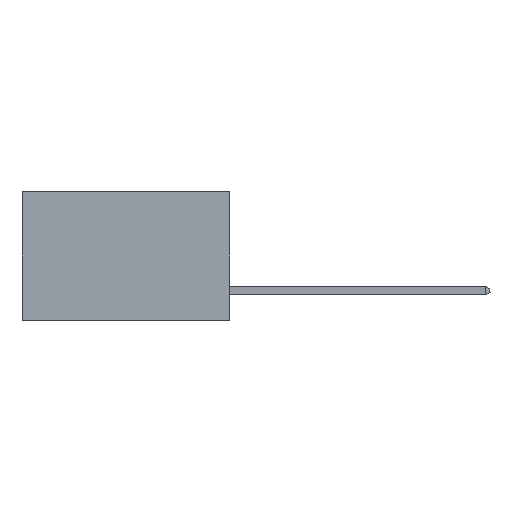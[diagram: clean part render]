
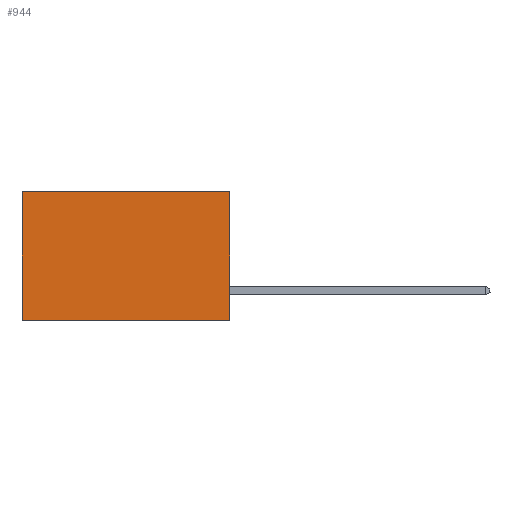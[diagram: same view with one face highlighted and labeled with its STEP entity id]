
A CAD part, left-side view. The second image highlights one B-rep face of the part: STEP entity #944.
In plain terms, the highlighted planar face has unit normal (-1, 0, 0).
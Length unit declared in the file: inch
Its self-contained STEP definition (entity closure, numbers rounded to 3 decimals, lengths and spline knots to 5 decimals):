
#235 = FACE_OUTER_BOUND ( 'NONE', #9415, .T. ) ;
#944 = ADVANCED_FACE ( 'NONE', ( #235 ), #9784, .F. ) ;
#2129 = VECTOR ( 'NONE', #9009, 39.37008 ) ;
#2631 = CARTESIAN_POINT ( 'NONE',  ( 0.298, 0., 0. ) ) ;
#3233 = ORIENTED_EDGE ( 'NONE', *, *, #7428, .F. ) ;
#3327 = VECTOR ( 'NONE', #15590, 39.37008 ) ;
#4082 = DIRECTION ( 'NONE',  ( 0., 1., 0. ) ) ;
#4445 = ORIENTED_EDGE ( 'NONE', *, *, #4800, .F. ) ;
#4634 = LINE ( 'NONE', #8909, #10448 ) ;
#4759 = VERTEX_POINT ( 'NONE', #16366 ) ;
#4800 = EDGE_CURVE ( 'NONE', #4759, #13359, #9547, .T. ) ;
#5524 = DIRECTION ( 'NONE',  ( 1., 0., 0. ) ) ;
#6224 = CARTESIAN_POINT ( 'NONE',  ( 0.298, 0.6, 0. ) ) ;
#7428 = EDGE_CURVE ( 'NONE', #13359, #11709, #4634, .T. ) ;
#7526 = VECTOR ( 'NONE', #4082, 39.37008 ) ;
#8736 = DIRECTION ( 'NONE',  ( 0., 1., 0. ) ) ;
#8909 = CARTESIAN_POINT ( 'NONE',  ( 0.298, 0., -0.37 ) ) ;
#9009 = DIRECTION ( 'NONE',  ( 0., 0., -1. ) ) ;
#9016 = CARTESIAN_POINT ( 'NONE',  ( 0.298, 0.6, -0.37 ) ) ;
#9415 = EDGE_LOOP ( 'NONE', ( #17513, #3233, #4445, #9582 ) ) ;
#9547 = LINE ( 'NONE', #17664, #2129 ) ;
#9582 = ORIENTED_EDGE ( 'NONE', *, *, #17725, .T. ) ;
#9784 = PLANE ( 'NONE',  #12416 ) ;
#10448 = VECTOR ( 'NONE', #8736, 39.37008 ) ;
#11709 = VERTEX_POINT ( 'NONE', #9016 ) ;
#12416 = AXIS2_PLACEMENT_3D ( 'NONE', #2631, #5524, #15574 ) ;
#13359 = VERTEX_POINT ( 'NONE', #17071 ) ;
#13582 = VERTEX_POINT ( 'NONE', #6224 ) ;
#15006 = LINE ( 'NONE', #15104, #3327 ) ;
#15104 = CARTESIAN_POINT ( 'NONE',  ( 0.298, 0.6, 0. ) ) ;
#15574 = DIRECTION ( 'NONE',  ( 0., 0., -1. ) ) ;
#15590 = DIRECTION ( 'NONE',  ( 0., 0., -1. ) ) ;
#15671 = EDGE_CURVE ( 'NONE', #13582, #11709, #15006, .T. ) ;
#16292 = LINE ( 'NONE', #16914, #7526 ) ;
#16366 = CARTESIAN_POINT ( 'NONE',  ( 0.298, 0., 0. ) ) ;
#16914 = CARTESIAN_POINT ( 'NONE',  ( 0.298, 0., 0. ) ) ;
#17071 = CARTESIAN_POINT ( 'NONE',  ( 0.298, 0., -0.37 ) ) ;
#17513 = ORIENTED_EDGE ( 'NONE', *, *, #15671, .T. ) ;
#17664 = CARTESIAN_POINT ( 'NONE',  ( 0.298, 0., 0. ) ) ;
#17725 = EDGE_CURVE ( 'NONE', #4759, #13582, #16292, .T. ) ;
